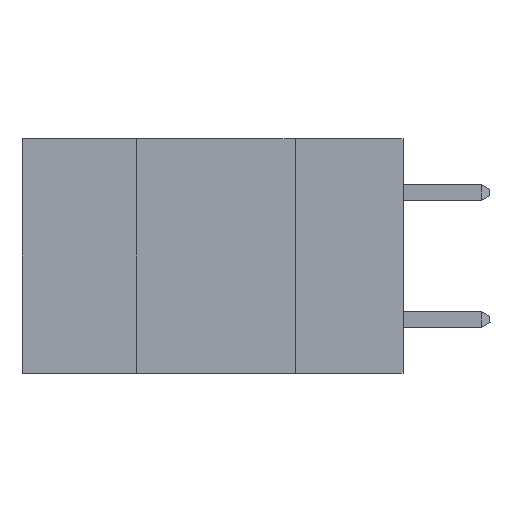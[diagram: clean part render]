
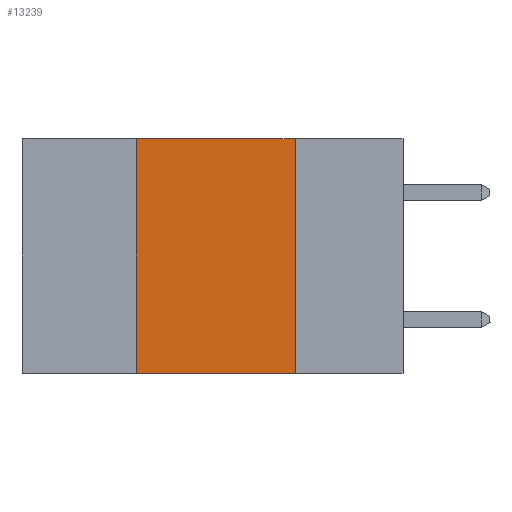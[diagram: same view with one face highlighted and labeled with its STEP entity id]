
A CAD part, left-side view. The second image highlights one B-rep face of the part: STEP entity #13239.
In plain terms, the highlighted planar face has unit normal (-1, 0, 0).
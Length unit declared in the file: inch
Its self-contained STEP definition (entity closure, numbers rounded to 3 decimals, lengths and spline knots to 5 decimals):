
#842 = VERTEX_POINT ( 'NONE', #10791 ) ;
#968 = VECTOR ( 'NONE', #1116, 39.37008 ) ;
#1104 = DIRECTION ( 'NONE',  ( 1., 0., 0. ) ) ;
#1116 = DIRECTION ( 'NONE',  ( 0., -1., 0. ) ) ;
#1553 = EDGE_CURVE ( 'NONE', #10269, #5156, #15444, .T. ) ;
#2425 = AXIS2_PLACEMENT_3D ( 'NONE', #10173, #1104, #11685 ) ;
#2500 = ORIENTED_EDGE ( 'NONE', *, *, #10708, .F. ) ;
#3514 = DIRECTION ( 'NONE',  ( 0., 0., 1. ) ) ;
#3837 = LINE ( 'NONE', #14107, #19336 ) ;
#3988 = EDGE_LOOP ( 'NONE', ( #18047, #2500, #6507, #18496 ) ) ;
#4533 = LINE ( 'NONE', #7037, #968 ) ;
#4818 = VERTEX_POINT ( 'NONE', #12540 ) ;
#5156 = VERTEX_POINT ( 'NONE', #5741 ) ;
#5741 = CARTESIAN_POINT ( 'NONE',  ( 0., 0.17, -0.37 ) ) ;
#6507 = ORIENTED_EDGE ( 'NONE', *, *, #16870, .F. ) ;
#7037 = CARTESIAN_POINT ( 'NONE',  ( 0., 0.6, -0.37 ) ) ;
#7305 = CARTESIAN_POINT ( 'NONE',  ( 0., 0.6, 0. ) ) ;
#8393 = LINE ( 'NONE', #7305, #11972 ) ;
#9454 = CARTESIAN_POINT ( 'NONE',  ( 0., 0.17, 0. ) ) ;
#10173 = CARTESIAN_POINT ( 'NONE',  ( 0., 0.6, 0. ) ) ;
#10235 = DIRECTION ( 'NONE',  ( 0., 0., -1. ) ) ;
#10269 = VERTEX_POINT ( 'NONE', #9454 ) ;
#10708 = EDGE_CURVE ( 'NONE', #842, #10269, #8393, .T. ) ;
#10791 = CARTESIAN_POINT ( 'NONE',  ( 0., 0.42, 0. ) ) ;
#11147 = FACE_OUTER_BOUND ( 'NONE', #3988, .T. ) ;
#11685 = DIRECTION ( 'NONE',  ( 0., 0., -1. ) ) ;
#11972 = VECTOR ( 'NONE', #16372, 39.37008 ) ;
#12540 = CARTESIAN_POINT ( 'NONE',  ( 0., 0.42, -0.37 ) ) ;
#13239 = ADVANCED_FACE ( 'NONE', ( #11147 ), #16160, .F. ) ;
#14107 = CARTESIAN_POINT ( 'NONE',  ( 0., 0.42, 0. ) ) ;
#14274 = EDGE_CURVE ( 'NONE', #4818, #5156, #4533, .T. ) ;
#14930 = CARTESIAN_POINT ( 'NONE',  ( 0., 0.17, 0. ) ) ;
#15444 = LINE ( 'NONE', #14930, #19370 ) ;
#16160 = PLANE ( 'NONE',  #2425 ) ;
#16372 = DIRECTION ( 'NONE',  ( 0., -1., 0. ) ) ;
#16870 = EDGE_CURVE ( 'NONE', #4818, #842, #3837, .T. ) ;
#18047 = ORIENTED_EDGE ( 'NONE', *, *, #1553, .F. ) ;
#18496 = ORIENTED_EDGE ( 'NONE', *, *, #14274, .T. ) ;
#19336 = VECTOR ( 'NONE', #3514, 39.37008 ) ;
#19370 = VECTOR ( 'NONE', #10235, 39.37008 ) ;
